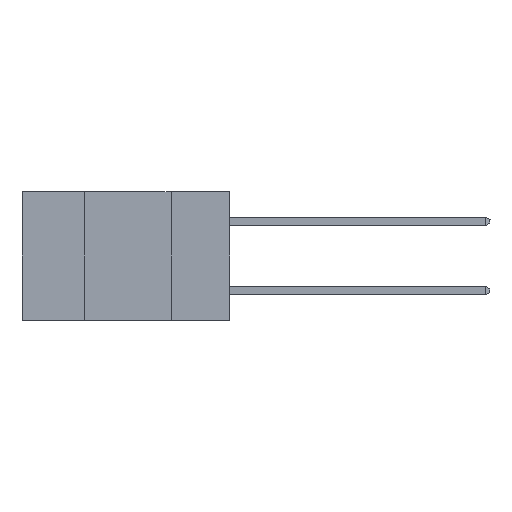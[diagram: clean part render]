
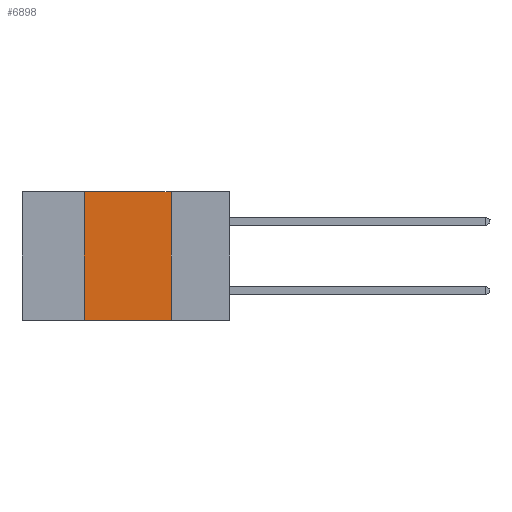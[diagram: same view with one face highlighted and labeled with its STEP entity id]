
A CAD part, left-side view. The second image highlights one B-rep face of the part: STEP entity #6898.
In plain terms, the highlighted planar face has unit normal (-1, 0, 0).
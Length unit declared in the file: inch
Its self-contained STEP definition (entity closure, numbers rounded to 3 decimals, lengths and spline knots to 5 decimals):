
#111 = ORIENTED_EDGE ( 'NONE', *, *, #22648, .F. ) ;
#2382 = CARTESIAN_POINT ( 'NONE',  ( 0., 0.42, 0. ) ) ;
#2633 = LINE ( 'NONE', #28504, #21211 ) ;
#3062 = EDGE_CURVE ( 'NONE', #23446, #29530, #2633, .T. ) ;
#3874 = CARTESIAN_POINT ( 'NONE',  ( 0., 0.17, 0. ) ) ;
#4357 = DIRECTION ( 'NONE',  ( 0., -1., 0. ) ) ;
#4729 = PLANE ( 'NONE',  #27619 ) ;
#5543 = LINE ( 'NONE', #29581, #19213 ) ;
#6898 = ADVANCED_FACE ( 'NONE', ( #14899 ), #4729, .F. ) ;
#7355 = DIRECTION ( 'NONE',  ( 1., 0., 0. ) ) ;
#8896 = EDGE_CURVE ( 'NONE', #25860, #29530, #5543, .T. ) ;
#8898 = EDGE_LOOP ( 'NONE', ( #27319, #23177, #111, #18771 ) ) ;
#8946 = CARTESIAN_POINT ( 'NONE',  ( 0., 0.6, 0. ) ) ;
#9646 = DIRECTION ( 'NONE',  ( 0., 0., -1. ) ) ;
#9745 = CARTESIAN_POINT ( 'NONE',  ( 0., 0.6, 0. ) ) ;
#11703 = EDGE_CURVE ( 'NONE', #29469, #25860, #27384, .T. ) ;
#14899 = FACE_OUTER_BOUND ( 'NONE', #8898, .T. ) ;
#15178 = CARTESIAN_POINT ( 'NONE',  ( 0., 0.42, 0. ) ) ;
#16684 = LINE ( 'NONE', #15178, #21981 ) ;
#18771 = ORIENTED_EDGE ( 'NONE', *, *, #3062, .T. ) ;
#19213 = VECTOR ( 'NONE', #19642, 39.37008 ) ;
#19642 = DIRECTION ( 'NONE',  ( 0., 0., -1. ) ) ;
#20815 = CARTESIAN_POINT ( 'NONE',  ( 0., 0.42, -0.37 ) ) ;
#21211 = VECTOR ( 'NONE', #4357, 39.37008 ) ;
#21981 = VECTOR ( 'NONE', #25089, 39.37008 ) ;
#22300 = CARTESIAN_POINT ( 'NONE',  ( 0., 0.17, -0.37 ) ) ;
#22648 = EDGE_CURVE ( 'NONE', #23446, #29469, #16684, .T. ) ;
#23177 = ORIENTED_EDGE ( 'NONE', *, *, #11703, .F. ) ;
#23446 = VERTEX_POINT ( 'NONE', #20815 ) ;
#23478 = DIRECTION ( 'NONE',  ( 0., -1., 0. ) ) ;
#25089 = DIRECTION ( 'NONE',  ( 0., 0., 1. ) ) ;
#25854 = VECTOR ( 'NONE', #23478, 39.37008 ) ;
#25860 = VERTEX_POINT ( 'NONE', #3874 ) ;
#27319 = ORIENTED_EDGE ( 'NONE', *, *, #8896, .F. ) ;
#27384 = LINE ( 'NONE', #8946, #25854 ) ;
#27619 = AXIS2_PLACEMENT_3D ( 'NONE', #9745, #7355, #9646 ) ;
#28504 = CARTESIAN_POINT ( 'NONE',  ( 0., 0.6, -0.37 ) ) ;
#29469 = VERTEX_POINT ( 'NONE', #2382 ) ;
#29530 = VERTEX_POINT ( 'NONE', #22300 ) ;
#29581 = CARTESIAN_POINT ( 'NONE',  ( 0., 0.17, 0. ) ) ;
